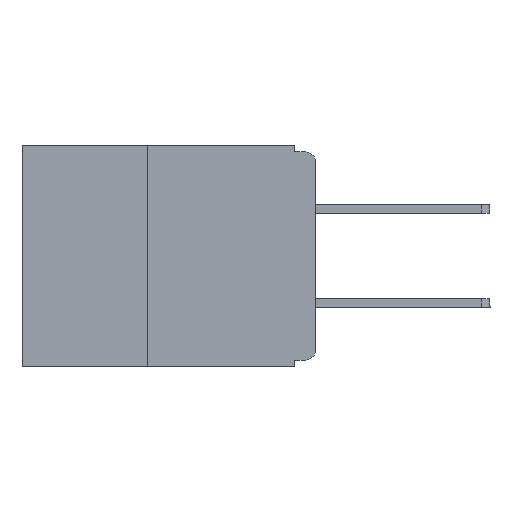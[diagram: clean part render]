
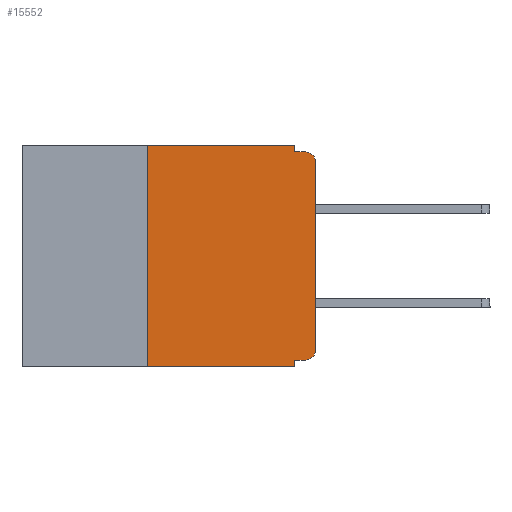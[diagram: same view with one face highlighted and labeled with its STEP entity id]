
A CAD part, left-side view. The second image highlights one B-rep face of the part: STEP entity #15552.
In plain terms, the highlighted planar face has unit normal (-1, 0, 0).
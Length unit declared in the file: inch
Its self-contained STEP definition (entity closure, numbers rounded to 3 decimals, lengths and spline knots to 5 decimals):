
#79 = FACE_OUTER_BOUND ( 'NONE', #7451, .T. ) ;
#516 = LINE ( 'NONE', #15816, #10447 ) ;
#812 = VECTOR ( 'NONE', #22088, 39.37008 ) ;
#927 = AXIS2_PLACEMENT_3D ( 'NONE', #20857, #17597, #7073 ) ;
#1040 = ORIENTED_EDGE ( 'NONE', *, *, #9926, .T. ) ;
#1194 = VERTEX_POINT ( 'NONE', #6085 ) ;
#1419 = CARTESIAN_POINT ( 'NONE',  ( 0., 0., 0. ) ) ;
#1438 = DIRECTION ( 'NONE',  ( 0., -1., 0. ) ) ;
#1579 = VERTEX_POINT ( 'NONE', #14408 ) ;
#1678 = VERTEX_POINT ( 'NONE', #22238 ) ;
#1781 = EDGE_CURVE ( 'NONE', #21893, #6061, #22449, .T. ) ;
#2604 = CARTESIAN_POINT ( 'NONE',  ( 0., 0.25, 0. ) ) ;
#3050 = DIRECTION ( 'NONE',  ( -1., 0., 0. ) ) ;
#3279 = AXIS2_PLACEMENT_3D ( 'NONE', #13768, #13763, #13736 ) ;
#3865 = ORIENTED_EDGE ( 'NONE', *, *, #6017, .F. ) ;
#3928 = LINE ( 'NONE', #17669, #17593 ) ;
#4000 = CARTESIAN_POINT ( 'NONE',  ( 0., 0.015, -0.01 ) ) ;
#4392 = ORIENTED_EDGE ( 'NONE', *, *, #5222, .T. ) ;
#4442 = DIRECTION ( 'NONE',  ( 0., 0., 1. ) ) ;
#4478 = VECTOR ( 'NONE', #17891, 39.37008 ) ;
#4563 = EDGE_CURVE ( 'NONE', #5830, #21893, #10680, .T. ) ;
#4598 = CARTESIAN_POINT ( 'NONE',  ( 0., 0.031, -0.01 ) ) ;
#4673 = CARTESIAN_POINT ( 'NONE',  ( 0., 0.25, -0.33 ) ) ;
#5097 = ORIENTED_EDGE ( 'NONE', *, *, #1781, .F. ) ;
#5146 = PLANE ( 'NONE',  #927 ) ;
#5222 = EDGE_CURVE ( 'NONE', #6820, #6061, #16166, .T. ) ;
#5428 = VERTEX_POINT ( 'NONE', #11560 ) ;
#5830 = VERTEX_POINT ( 'NONE', #6421 ) ;
#6017 = EDGE_CURVE ( 'NONE', #5428, #19157, #18232, .T. ) ;
#6061 = VERTEX_POINT ( 'NONE', #4000 ) ;
#6085 = CARTESIAN_POINT ( 'NONE',  ( 0., 0.031, -0.33 ) ) ;
#6421 = CARTESIAN_POINT ( 'NONE',  ( 0., 0.031, 0. ) ) ;
#6701 = VERTEX_POINT ( 'NONE', #18897 ) ;
#6820 = VERTEX_POINT ( 'NONE', #15912 ) ;
#6839 = EDGE_CURVE ( 'NONE', #6701, #6820, #11156, .T. ) ;
#7073 = DIRECTION ( 'NONE',  ( 0., 0., -1. ) ) ;
#7379 = CARTESIAN_POINT ( 'NONE',  ( 0., 0., -0.32 ) ) ;
#7451 = EDGE_LOOP ( 'NONE', ( #13256, #4392, #5097, #22006, #11856, #3865, #1040, #16917, #10618, #14532 ) ) ;
#7991 = LINE ( 'NONE', #17915, #21165 ) ;
#9571 = VECTOR ( 'NONE', #4442, 39.37008 ) ;
#9926 = EDGE_CURVE ( 'NONE', #5428, #1194, #3928, .T. ) ;
#10447 = VECTOR ( 'NONE', #10493, 39.37008 ) ;
#10493 = DIRECTION ( 'NONE',  ( 0., 0., -1. ) ) ;
#10577 = VECTOR ( 'NONE', #15980, 39.37008 ) ;
#10618 = ORIENTED_EDGE ( 'NONE', *, *, #12801, .F. ) ;
#10680 = LINE ( 'NONE', #22119, #812 ) ;
#10979 = AXIS2_PLACEMENT_3D ( 'NONE', #13960, #3050, #15720 ) ;
#11156 = LINE ( 'NONE', #1419, #10577 ) ;
#11560 = CARTESIAN_POINT ( 'NONE',  ( 0., 0.25, -0.33 ) ) ;
#11856 = ORIENTED_EDGE ( 'NONE', *, *, #21553, .F. ) ;
#12073 = VECTOR ( 'NONE', #19533, 39.37008 ) ;
#12801 = EDGE_CURVE ( 'NONE', #1678, #1579, #21092, .T. ) ;
#13256 = ORIENTED_EDGE ( 'NONE', *, *, #6839, .T. ) ;
#13736 = DIRECTION ( 'NONE',  ( 0., 0., -1. ) ) ;
#13763 = DIRECTION ( 'NONE',  ( -1., 0., 0. ) ) ;
#13768 = CARTESIAN_POINT ( 'NONE',  ( 0., 0.015, -0.025 ) ) ;
#13960 = CARTESIAN_POINT ( 'NONE',  ( 0., 0.015, -0.305 ) ) ;
#14408 = CARTESIAN_POINT ( 'NONE',  ( 0., 0.031, -0.32 ) ) ;
#14532 = ORIENTED_EDGE ( 'NONE', *, *, #21976, .T. ) ;
#15552 = ADVANCED_FACE ( 'NONE', ( #79 ), #5146, .F. ) ;
#15720 = DIRECTION ( 'NONE',  ( 0., 0., -1. ) ) ;
#15816 = CARTESIAN_POINT ( 'NONE',  ( 0., 0.031, -0.33 ) ) ;
#15912 = CARTESIAN_POINT ( 'NONE',  ( 0., 0., -0.025 ) ) ;
#15980 = DIRECTION ( 'NONE',  ( 0., 0., 1. ) ) ;
#16166 = CIRCLE ( 'NONE', #3279, 0.015 ) ;
#16917 = ORIENTED_EDGE ( 'NONE', *, *, #19309, .F. ) ;
#17593 = VECTOR ( 'NONE', #1438, 39.37008 ) ;
#17597 = DIRECTION ( 'NONE',  ( 1., 0., 0. ) ) ;
#17669 = CARTESIAN_POINT ( 'NONE',  ( 0., 0.437, -0.33 ) ) ;
#17891 = DIRECTION ( 'NONE',  ( 0., -1., 0. ) ) ;
#17915 = CARTESIAN_POINT ( 'NONE',  ( 0., 0.437, 0. ) ) ;
#18232 = LINE ( 'NONE', #4673, #9571 ) ;
#18897 = CARTESIAN_POINT ( 'NONE',  ( 0., 0., -0.305 ) ) ;
#19157 = VERTEX_POINT ( 'NONE', #2604 ) ;
#19309 = EDGE_CURVE ( 'NONE', #1579, #1194, #516, .T. ) ;
#19533 = DIRECTION ( 'NONE',  ( 0., 1., 0. ) ) ;
#20632 = CIRCLE ( 'NONE', #10979, 0.015 ) ;
#20857 = CARTESIAN_POINT ( 'NONE',  ( 0., 0.437, 0. ) ) ;
#21092 = LINE ( 'NONE', #7379, #12073 ) ;
#21165 = VECTOR ( 'NONE', #22773, 39.37008 ) ;
#21553 = EDGE_CURVE ( 'NONE', #19157, #5830, #7991, .T. ) ;
#21893 = VERTEX_POINT ( 'NONE', #4598 ) ;
#21976 = EDGE_CURVE ( 'NONE', #1678, #6701, #20632, .T. ) ;
#22006 = ORIENTED_EDGE ( 'NONE', *, *, #4563, .F. ) ;
#22088 = DIRECTION ( 'NONE',  ( 0., 0., -1. ) ) ;
#22119 = CARTESIAN_POINT ( 'NONE',  ( 0., 0.031, 0. ) ) ;
#22238 = CARTESIAN_POINT ( 'NONE',  ( 0., 0.015, -0.32 ) ) ;
#22449 = LINE ( 'NONE', #22636, #4478 ) ;
#22636 = CARTESIAN_POINT ( 'NONE',  ( 0., 0., -0.01 ) ) ;
#22773 = DIRECTION ( 'NONE',  ( 0., -1., 0. ) ) ;
